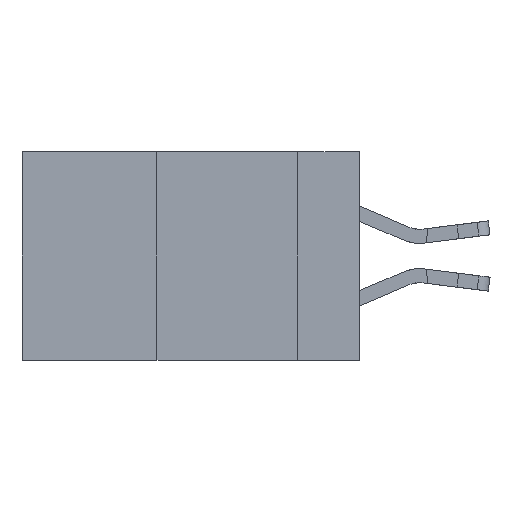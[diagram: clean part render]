
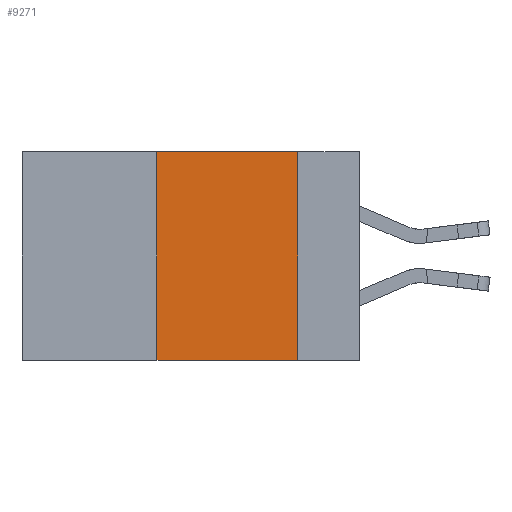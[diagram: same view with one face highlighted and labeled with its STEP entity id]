
A CAD part, left-side view. The second image highlights one B-rep face of the part: STEP entity #9271.
In plain terms, the highlighted planar face has unit normal (-1, 0, 0).
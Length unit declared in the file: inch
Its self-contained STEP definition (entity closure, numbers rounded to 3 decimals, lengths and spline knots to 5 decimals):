
#933 = LINE ( 'NONE', #19398, #13351 ) ;
#1271 = VERTEX_POINT ( 'NONE', #10166 ) ;
#1618 = CARTESIAN_POINT ( 'NONE',  ( 0., 0.6, 0. ) ) ;
#2526 = FACE_OUTER_BOUND ( 'NONE', #11402, .T. ) ;
#2689 = ORIENTED_EDGE ( 'NONE', *, *, #20687, .F. ) ;
#2941 = EDGE_CURVE ( 'NONE', #8621, #11306, #3061, .T. ) ;
#3061 = LINE ( 'NONE', #11354, #8896 ) ;
#3801 = VERTEX_POINT ( 'NONE', #15313 ) ;
#4351 = DIRECTION ( 'NONE',  ( 0., 0., -1. ) ) ;
#4476 = EDGE_CURVE ( 'NONE', #1271, #3801, #933, .T. ) ;
#4818 = DIRECTION ( 'NONE',  ( 0., 0., -1. ) ) ;
#6623 = ORIENTED_EDGE ( 'NONE', *, *, #2941, .F. ) ;
#6631 = DIRECTION ( 'NONE',  ( 0., -1., 0. ) ) ;
#6656 = EDGE_CURVE ( 'NONE', #1271, #8621, #19293, .T. ) ;
#7177 = VECTOR ( 'NONE', #4351, 39.37008 ) ;
#7519 = ORIENTED_EDGE ( 'NONE', *, *, #6656, .F. ) ;
#8621 = VERTEX_POINT ( 'NONE', #20976 ) ;
#8896 = VECTOR ( 'NONE', #11547, 39.37008 ) ;
#9271 = ADVANCED_FACE ( 'NONE', ( #2526 ), #14779, .F. ) ;
#9357 = DIRECTION ( 'NONE',  ( 0., 0., 1. ) ) ;
#9912 = DIRECTION ( 'NONE',  ( 1., 0., 0. ) ) ;
#10166 = CARTESIAN_POINT ( 'NONE',  ( 0., 0.36, -0.37 ) ) ;
#11306 = VERTEX_POINT ( 'NONE', #14029 ) ;
#11354 = CARTESIAN_POINT ( 'NONE',  ( 0., 0.6, 0. ) ) ;
#11402 = EDGE_LOOP ( 'NONE', ( #2689, #6623, #7519, #17208 ) ) ;
#11547 = DIRECTION ( 'NONE',  ( 0., -1., 0. ) ) ;
#13351 = VECTOR ( 'NONE', #6631, 39.37008 ) ;
#13477 = VECTOR ( 'NONE', #9357, 39.37008 ) ;
#14019 = CARTESIAN_POINT ( 'NONE',  ( 0., 0.11, 0. ) ) ;
#14029 = CARTESIAN_POINT ( 'NONE',  ( 0., 0.11, 0. ) ) ;
#14779 = PLANE ( 'NONE',  #20103 ) ;
#15313 = CARTESIAN_POINT ( 'NONE',  ( 0., 0.11, -0.37 ) ) ;
#17063 = LINE ( 'NONE', #14019, #7177 ) ;
#17208 = ORIENTED_EDGE ( 'NONE', *, *, #4476, .T. ) ;
#19293 = LINE ( 'NONE', #20442, #13477 ) ;
#19398 = CARTESIAN_POINT ( 'NONE',  ( 0., 0.6, -0.37 ) ) ;
#20103 = AXIS2_PLACEMENT_3D ( 'NONE', #1618, #9912, #4818 ) ;
#20442 = CARTESIAN_POINT ( 'NONE',  ( 0., 0.36, 0. ) ) ;
#20687 = EDGE_CURVE ( 'NONE', #11306, #3801, #17063, .T. ) ;
#20976 = CARTESIAN_POINT ( 'NONE',  ( 0., 0.36, 0. ) ) ;
